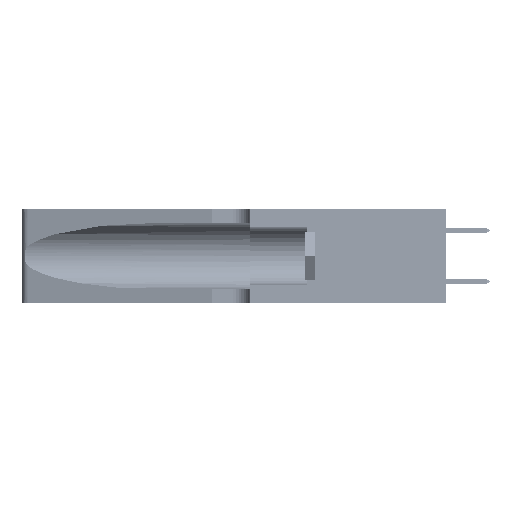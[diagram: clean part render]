
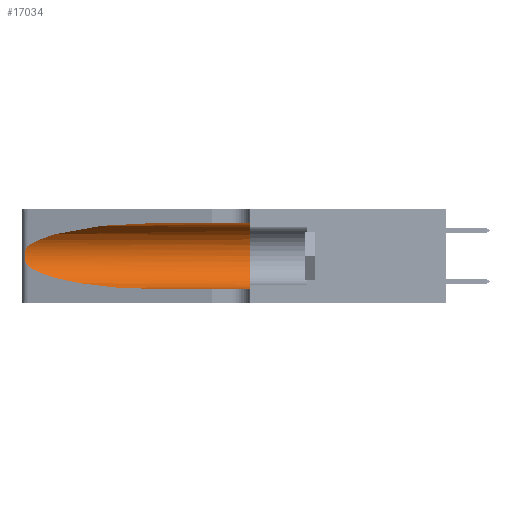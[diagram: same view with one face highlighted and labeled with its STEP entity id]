
A CAD part, left-side view. The second image highlights one B-rep face of the part: STEP entity #17034.
In plain terms, the highlighted cylindrical face has radius 3.308 mm (diameter 6.617 mm), a partial arc.
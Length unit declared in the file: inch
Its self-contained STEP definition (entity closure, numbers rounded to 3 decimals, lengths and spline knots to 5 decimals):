
#30 = VERTEX_POINT ( 'NONE', #4798 ) ;
#2166 = B_SPLINE_CURVE_WITH_KNOTS ( 'NONE', 3,
 ( #18968, #52136, #31473, #6719, #35655, #10872, #39807, #14999, #43961, #19150, #48138, #23340, #52317, #27489 ),
 .UNSPECIFIED., .F., .F.,
 ( 4, 2, 2, 2, 2, 2, 4 ),
 ( 0., 0.00027, 0.00053, 0.00107, 0.0016, 0.00187, 0.00214 ),
 .UNSPECIFIED. ) ;
#2838 = EDGE_CURVE ( 'NONE', #45552, #33600, #4566, .T. ) ;
#3051 = CIRCLE ( 'NONE', #10705, 0.13025 ) ;
#3279 = EDGE_CURVE ( 'NONE', #47908, #45679, #2166, .T. ) ;
#3694 = DIRECTION ( 'NONE',  ( 0., 1., 0. ) ) ;
#4566 = LINE ( 'NONE', #52132, #49888 ) ;
#4798 = CARTESIAN_POINT ( 'NONE',  ( 0.1305, 0.35, 0.05475 ) ) ;
#6719 = CARTESIAN_POINT ( 'NONE',  ( 0.25787, 1.23484, 0.2124 ) ) ;
#6732 = EDGE_CURVE ( 'NONE', #45552, #47908, #20290, .T. ) ;
#8445 = EDGE_CURVE ( 'NONE', #45679, #25444, #44886, .T. ) ;
#9197 = EDGE_CURVE ( 'NONE', #33600, #30, #3051, .T. ) ;
#10705 = AXIS2_PLACEMENT_3D ( 'NONE', #28451, #3694, #32600 ) ;
#10872 = CARTESIAN_POINT ( 'NONE',  ( 0.26018, 1.23835, 0.19895 ) ) ;
#10962 = CARTESIAN_POINT ( 'NONE',  ( 0.1305, 0.35, 0.31525 ) ) ;
#10979 = CARTESIAN_POINT ( 'NONE',  ( 0.2373, 1.15595, 0.08982 ) ) ;
#13284 = CARTESIAN_POINT ( 'NONE',  ( 0.25487, 1.22718, 0.22369 ) ) ;
#14732 = ORIENTED_EDGE ( 'NONE', *, *, #9197, .F. ) ;
#14999 = CARTESIAN_POINT ( 'NONE',  ( 0.26075, 1.23896, 0.178 ) ) ;
#15113 = CARTESIAN_POINT ( 'NONE',  ( 0.1305, 0.72297, 0.05475 ) ) ;
#17034 = ADVANCED_FACE ( 'NONE', ( #18300 ), #28015, .F. ) ;
#17253 = CARTESIAN_POINT ( 'NONE',  ( 0.18966, 0.96281, 0.31525 ) ) ;
#18300 = FACE_OUTER_BOUND ( 'NONE', #44945, .T. ) ;
#18886 = CARTESIAN_POINT ( 'NONE',  ( 0.25487, 1.22718, 0.22369 ) ) ;
#18968 = CARTESIAN_POINT ( 'NONE',  ( 0.25487, 1.22718, 0.22369 ) ) ;
#19150 = CARTESIAN_POINT ( 'NONE',  ( 0.25856, 1.23593, 0.16098 ) ) ;
#19181 = VECTOR ( 'NONE', #21208, 39.37008 ) ;
#20290 =( BOUNDED_CURVE ( )  B_SPLINE_CURVE ( 3, ( #38055, #17253, #33906, #13284 ),
 .UNSPECIFIED., .F., .F. ) 
 B_SPLINE_CURVE_WITH_KNOTS ( ( 4, 4 ),
 ( 1.5708, 2.84003 ),
 .UNSPECIFIED. ) 
 CURVE ( )  GEOMETRIC_REPRESENTATION_ITEM ( )  RATIONAL_B_SPLINE_CURVE ( ( 1., 0.87, 0.87, 1. ) ) 
 REPRESENTATION_ITEM ( '' )  );
#20349 = CARTESIAN_POINT ( 'NONE',  ( 0.25487, 1.22718, 0.14631 ) ) ;
#20557 = CARTESIAN_POINT ( 'NONE',  ( 0.1305, 0.72297, 0.05475 ) ) ;
#21208 = DIRECTION ( 'NONE',  ( 0., -1., 0. ) ) ;
#21689 = CARTESIAN_POINT ( 'NONE',  ( 0.1305, 1.61858, 0.185 ) ) ;
#23340 = CARTESIAN_POINT ( 'NONE',  ( 0.25639, 1.23186, 0.15144 ) ) ;
#24187 = ORIENTED_EDGE ( 'NONE', *, *, #6732, .T. ) ;
#25360 = CARTESIAN_POINT ( 'NONE',  ( 0.1305, 1.61858, 0.05475 ) ) ;
#25444 = VERTEX_POINT ( 'NONE', #20557 ) ;
#25836 = DIRECTION ( 'NONE',  ( 0., 0., -1. ) ) ;
#27300 = DIRECTION ( 'NONE',  ( 0., -1., 0. ) ) ;
#27489 = CARTESIAN_POINT ( 'NONE',  ( 0.25487, 1.22718, 0.14631 ) ) ;
#28015 = CYLINDRICAL_SURFACE ( 'NONE', #47593, 0.13025 ) ;
#28451 = CARTESIAN_POINT ( 'NONE',  ( 0.1305, 0.35, 0.185 ) ) ;
#29541 = ORIENTED_EDGE ( 'NONE', *, *, #41676, .T. ) ;
#30212 = LINE ( 'NONE', #25360, #19181 ) ;
#31473 = CARTESIAN_POINT ( 'NONE',  ( 0.25639, 1.23184, 0.21858 ) ) ;
#31579 = CARTESIAN_POINT ( 'NONE',  ( 0.18966, 0.96281, 0.05475 ) ) ;
#32600 = DIRECTION ( 'NONE',  ( 0., 0., 1. ) ) ;
#33209 = ORIENTED_EDGE ( 'NONE', *, *, #2838, .F. ) ;
#33600 = VERTEX_POINT ( 'NONE', #10962 ) ;
#33906 = CARTESIAN_POINT ( 'NONE',  ( 0.2373, 1.15595, 0.28018 ) ) ;
#35655 = CARTESIAN_POINT ( 'NONE',  ( 0.25854, 1.2359, 0.20912 ) ) ;
#35921 = CARTESIAN_POINT ( 'NONE',  ( 0.1305, 0.72297, 0.31525 ) ) ;
#37879 = ORIENTED_EDGE ( 'NONE', *, *, #3279, .T. ) ;
#38055 = CARTESIAN_POINT ( 'NONE',  ( 0.1305, 0.72297, 0.31525 ) ) ;
#38129 = DIRECTION ( 'NONE',  ( 0., -1., 0. ) ) ;
#39807 = CARTESIAN_POINT ( 'NONE',  ( 0.26075, 1.23896, 0.19203 ) ) ;
#39912 = CARTESIAN_POINT ( 'NONE',  ( 0.25487, 1.22718, 0.14631 ) ) ;
#41676 = EDGE_CURVE ( 'NONE', #25444, #30, #30212, .T. ) ;
#43961 = CARTESIAN_POINT ( 'NONE',  ( 0.26017, 1.23833, 0.17102 ) ) ;
#44886 =( BOUNDED_CURVE ( )  B_SPLINE_CURVE ( 3, ( #39912, #10979, #31579, #15113 ),
 .UNSPECIFIED., .F., .T. ) 
 B_SPLINE_CURVE_WITH_KNOTS ( ( 4, 4 ),
 ( 3.44316, 4.71239 ),
 .UNSPECIFIED. ) 
 CURVE ( )  GEOMETRIC_REPRESENTATION_ITEM ( )  RATIONAL_B_SPLINE_CURVE ( ( 1., 0.87, 0.87, 1. ) ) 
 REPRESENTATION_ITEM ( '' )  );
#44945 = EDGE_LOOP ( 'NONE', ( #24187, #37879, #49724, #29541, #14732, #33209 ) ) ;
#45552 = VERTEX_POINT ( 'NONE', #35921 ) ;
#45679 = VERTEX_POINT ( 'NONE', #20349 ) ;
#47593 = AXIS2_PLACEMENT_3D ( 'NONE', #21689, #38129, #25836 ) ;
#47908 = VERTEX_POINT ( 'NONE', #18886 ) ;
#48138 = CARTESIAN_POINT ( 'NONE',  ( 0.25789, 1.23486, 0.15765 ) ) ;
#49724 = ORIENTED_EDGE ( 'NONE', *, *, #8445, .T. ) ;
#49888 = VECTOR ( 'NONE', #27300, 39.37008 ) ;
#52132 = CARTESIAN_POINT ( 'NONE',  ( 0.1305, 1.61858, 0.31525 ) ) ;
#52136 = CARTESIAN_POINT ( 'NONE',  ( 0.25555, 1.22994, 0.2215 ) ) ;
#52317 = CARTESIAN_POINT ( 'NONE',  ( 0.25555, 1.22993, 0.14849 ) ) ;
